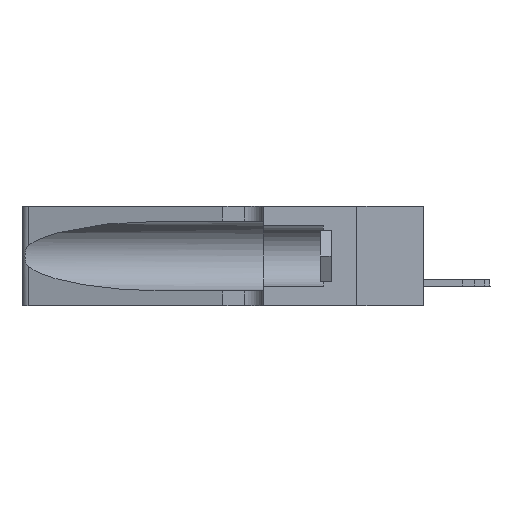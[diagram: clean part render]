
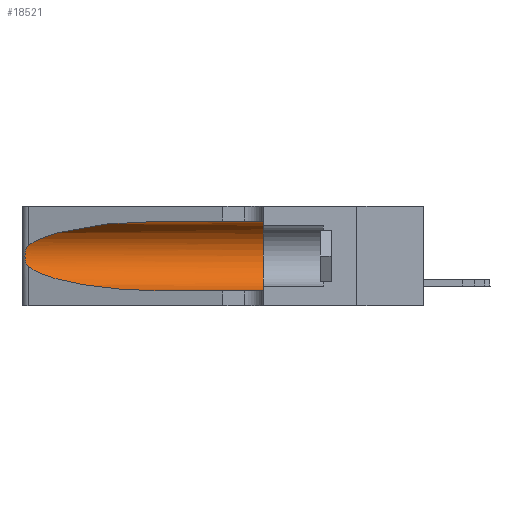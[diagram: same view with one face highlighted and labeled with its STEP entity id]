
A CAD part, left-side view. The second image highlights one B-rep face of the part: STEP entity #18521.
In plain terms, the highlighted cylindrical face has radius 3.308 mm (diameter 6.617 mm), a partial arc.
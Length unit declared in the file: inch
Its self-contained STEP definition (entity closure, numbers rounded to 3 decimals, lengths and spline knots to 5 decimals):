
#37 = CARTESIAN_POINT ( 'NONE',  ( 0.25487, 1.22718, 0.22369 ) ) ;
#577 = LINE ( 'NONE', #21830, #1016 ) ;
#709 = CARTESIAN_POINT ( 'NONE',  ( 0.25789, 1.23486, 0.15765 ) ) ;
#834 = CARTESIAN_POINT ( 'NONE',  ( 0.25555, 1.22993, 0.14849 ) ) ;
#1016 = VECTOR ( 'NONE', #19833, 39.37008 ) ;
#1577 = EDGE_CURVE ( 'NONE', #33250, #14445, #26934, .T. ) ;
#2957 = CARTESIAN_POINT ( 'NONE',  ( 0.25555, 1.22994, 0.2215 ) ) ;
#3283 = CARTESIAN_POINT ( 'NONE',  ( 0.1305, 0.72297, 0.31525 ) ) ;
#3598 = CARTESIAN_POINT ( 'NONE',  ( 0.1305, 1.61858, 0.05475 ) ) ;
#3726 = EDGE_CURVE ( 'NONE', #27988, #21044, #28491, .T. ) ;
#5335 = CARTESIAN_POINT ( 'NONE',  ( 0.1305, 0.72297, 0.31525 ) ) ;
#5491 = FACE_OUTER_BOUND ( 'NONE', #8835, .T. ) ;
#5662 = EDGE_CURVE ( 'NONE', #32470, #27988, #20267, .T. ) ;
#6017 = CARTESIAN_POINT ( 'NONE',  ( 0.25787, 1.23484, 0.2124 ) ) ;
#6550 = DIRECTION ( 'NONE',  ( 0., 0., 1. ) ) ;
#6931 = ORIENTED_EDGE ( 'NONE', *, *, #3726, .T. ) ;
#8835 = EDGE_LOOP ( 'NONE', ( #25399, #26504, #23959, #6931, #22490, #27556 ) ) ;
#11561 = EDGE_CURVE ( 'NONE', #14445, #32470, #14026, .T. ) ;
#13091 = CARTESIAN_POINT ( 'NONE',  ( 0.1305, 0.72297, 0.05475 ) ) ;
#13376 = CARTESIAN_POINT ( 'NONE',  ( 0.2373, 1.15595, 0.08982 ) ) ;
#14026 = B_SPLINE_CURVE_WITH_KNOTS ( 'NONE', 3,
 ( #26837, #2957, #27295, #6017, #30294, #14175, #18970, #29824, #22626, #25280, #709, #28041, #834, #19552 ),
 .UNSPECIFIED., .F., .F.,
 ( 4, 2, 2, 2, 2, 2, 4 ),
 ( 0., 0.00027, 0.00053, 0.00107, 0.0016, 0.00187, 0.00214 ),
 .UNSPECIFIED. ) ;
#14175 = CARTESIAN_POINT ( 'NONE',  ( 0.26018, 1.23835, 0.19895 ) ) ;
#14445 = VERTEX_POINT ( 'NONE', #27665 ) ;
#14711 = DIRECTION ( 'NONE',  ( 0., 0., -1. ) ) ;
#16197 = CARTESIAN_POINT ( 'NONE',  ( 0.18966, 0.96281, 0.31525 ) ) ;
#17173 = DIRECTION ( 'NONE',  ( 0., -1., 0. ) ) ;
#17613 = CIRCLE ( 'NONE', #21039, 0.13025 ) ;
#18521 = ADVANCED_FACE ( 'NONE', ( #5491 ), #19366, .F. ) ;
#18867 = CARTESIAN_POINT ( 'NONE',  ( 0.2373, 1.15595, 0.28018 ) ) ;
#18970 = CARTESIAN_POINT ( 'NONE',  ( 0.26075, 1.23896, 0.19203 ) ) ;
#19366 = CYLINDRICAL_SURFACE ( 'NONE', #25168, 0.13025 ) ;
#19552 = CARTESIAN_POINT ( 'NONE',  ( 0.25487, 1.22718, 0.14631 ) ) ;
#19731 = CARTESIAN_POINT ( 'NONE',  ( 0.1305, 0.35, 0.05475 ) ) ;
#19833 = DIRECTION ( 'NONE',  ( 0., -1., 0. ) ) ;
#19954 = CARTESIAN_POINT ( 'NONE',  ( 0.1305, 0.35, 0.185 ) ) ;
#20267 =( BOUNDED_CURVE ( )  B_SPLINE_CURVE ( 3, ( #29474, #13376, #21225, #32199 ),
 .UNSPECIFIED., .F., .T. ) 
 B_SPLINE_CURVE_WITH_KNOTS ( ( 4, 4 ),
 ( 3.44316, 4.71239 ),
 .UNSPECIFIED. ) 
 CURVE ( )  GEOMETRIC_REPRESENTATION_ITEM ( )  RATIONAL_B_SPLINE_CURVE ( ( 1., 0.87, 0.87, 1. ) ) 
 REPRESENTATION_ITEM ( '' )  );
#21039 = AXIS2_PLACEMENT_3D ( 'NONE', #19954, #25451, #6550 ) ;
#21044 = VERTEX_POINT ( 'NONE', #19731 ) ;
#21225 = CARTESIAN_POINT ( 'NONE',  ( 0.18966, 0.96281, 0.05475 ) ) ;
#21830 = CARTESIAN_POINT ( 'NONE',  ( 0.1305, 1.61858, 0.31525 ) ) ;
#22490 = ORIENTED_EDGE ( 'NONE', *, *, #33906, .F. ) ;
#22577 = VECTOR ( 'NONE', #17173, 39.37008 ) ;
#22626 = CARTESIAN_POINT ( 'NONE',  ( 0.26017, 1.23833, 0.17102 ) ) ;
#23959 = ORIENTED_EDGE ( 'NONE', *, *, #5662, .T. ) ;
#25168 = AXIS2_PLACEMENT_3D ( 'NONE', #28083, #25449, #14711 ) ;
#25280 = CARTESIAN_POINT ( 'NONE',  ( 0.25856, 1.23593, 0.16098 ) ) ;
#25399 = ORIENTED_EDGE ( 'NONE', *, *, #1577, .T. ) ;
#25449 = DIRECTION ( 'NONE',  ( 0., -1., 0. ) ) ;
#25451 = DIRECTION ( 'NONE',  ( 0., 1., 0. ) ) ;
#26504 = ORIENTED_EDGE ( 'NONE', *, *, #11561, .T. ) ;
#26837 = CARTESIAN_POINT ( 'NONE',  ( 0.25487, 1.22718, 0.22369 ) ) ;
#26934 =( BOUNDED_CURVE ( )  B_SPLINE_CURVE ( 3, ( #5335, #16197, #18867, #37 ),
 .UNSPECIFIED., .F., .F. ) 
 B_SPLINE_CURVE_WITH_KNOTS ( ( 4, 4 ),
 ( 1.5708, 2.84003 ),
 .UNSPECIFIED. ) 
 CURVE ( )  GEOMETRIC_REPRESENTATION_ITEM ( )  RATIONAL_B_SPLINE_CURVE ( ( 1., 0.87, 0.87, 1. ) ) 
 REPRESENTATION_ITEM ( '' )  );
#27295 = CARTESIAN_POINT ( 'NONE',  ( 0.25639, 1.23184, 0.21858 ) ) ;
#27556 = ORIENTED_EDGE ( 'NONE', *, *, #29306, .F. ) ;
#27665 = CARTESIAN_POINT ( 'NONE',  ( 0.25487, 1.22718, 0.22369 ) ) ;
#27988 = VERTEX_POINT ( 'NONE', #13091 ) ;
#28041 = CARTESIAN_POINT ( 'NONE',  ( 0.25639, 1.23186, 0.15144 ) ) ;
#28083 = CARTESIAN_POINT ( 'NONE',  ( 0.1305, 1.61858, 0.185 ) ) ;
#28491 = LINE ( 'NONE', #3598, #22577 ) ;
#29306 = EDGE_CURVE ( 'NONE', #33250, #31413, #577, .T. ) ;
#29474 = CARTESIAN_POINT ( 'NONE',  ( 0.25487, 1.22718, 0.14631 ) ) ;
#29824 = CARTESIAN_POINT ( 'NONE',  ( 0.26075, 1.23896, 0.178 ) ) ;
#30294 = CARTESIAN_POINT ( 'NONE',  ( 0.25854, 1.2359, 0.20912 ) ) ;
#31413 = VERTEX_POINT ( 'NONE', #33229 ) ;
#32199 = CARTESIAN_POINT ( 'NONE',  ( 0.1305, 0.72297, 0.05475 ) ) ;
#32207 = CARTESIAN_POINT ( 'NONE',  ( 0.25487, 1.22718, 0.14631 ) ) ;
#32470 = VERTEX_POINT ( 'NONE', #32207 ) ;
#33229 = CARTESIAN_POINT ( 'NONE',  ( 0.1305, 0.35, 0.31525 ) ) ;
#33250 = VERTEX_POINT ( 'NONE', #3283 ) ;
#33906 = EDGE_CURVE ( 'NONE', #31413, #21044, #17613, .T. ) ;
